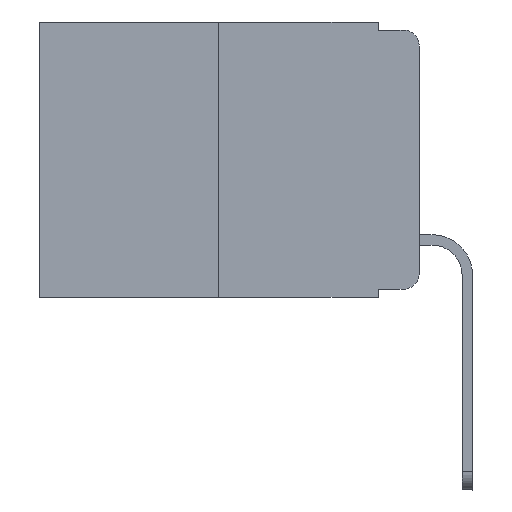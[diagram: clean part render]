
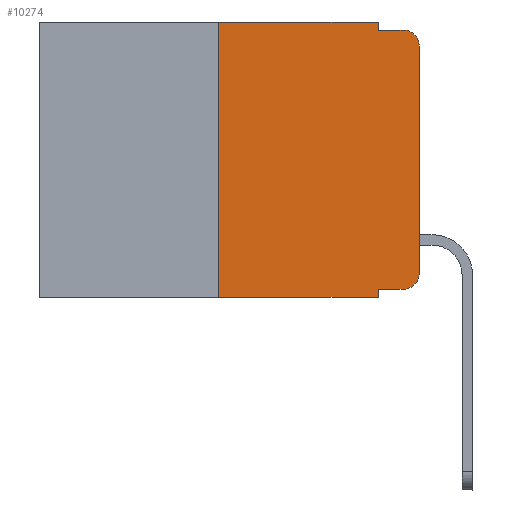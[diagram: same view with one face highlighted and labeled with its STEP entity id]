
A CAD part, left-side view. The second image highlights one B-rep face of the part: STEP entity #10274.
In plain terms, the highlighted planar face has unit normal (-1, 0, 0).
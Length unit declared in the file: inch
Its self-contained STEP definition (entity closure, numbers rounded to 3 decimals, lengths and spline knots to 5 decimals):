
#385 = EDGE_CURVE ( 'NONE', #6108, #2587, #17679, .T. ) ;
#498 = DIRECTION ( 'NONE',  ( 0., -1., 0. ) ) ;
#574 = DIRECTION ( 'NONE',  ( 0., 0., -1. ) ) ;
#698 = DIRECTION ( 'NONE',  ( 0., 0., -1. ) ) ;
#1213 = CARTESIAN_POINT ( 'NONE',  ( 0., 0.25, 0. ) ) ;
#1419 = LINE ( 'NONE', #10038, #11626 ) ;
#1794 = AXIS2_PLACEMENT_3D ( 'NONE', #13745, #10704, #574 ) ;
#1986 = FACE_OUTER_BOUND ( 'NONE', #2084, .T. ) ;
#2084 = EDGE_LOOP ( 'NONE', ( #8032, #12121, #10977, #15639, #12197, #11485, #10493, #4120, #3151, #17643 ) ) ;
#2191 = CARTESIAN_POINT ( 'NONE',  ( 0., 0.02, -0.313 ) ) ;
#2426 = AXIS2_PLACEMENT_3D ( 'NONE', #2191, #8846, #7192 ) ;
#2587 = VERTEX_POINT ( 'NONE', #17947 ) ;
#2642 = EDGE_CURVE ( 'NONE', #7393, #19901, #13010, .T. ) ;
#3125 = VERTEX_POINT ( 'NONE', #9799 ) ;
#3151 = ORIENTED_EDGE ( 'NONE', *, *, #16455, .T. ) ;
#3182 = CARTESIAN_POINT ( 'NONE',  ( 0., 0.051, 0. ) ) ;
#3537 = VECTOR ( 'NONE', #4506, 39.37008 ) ;
#3966 = VECTOR ( 'NONE', #498, 39.37008 ) ;
#4120 = ORIENTED_EDGE ( 'NONE', *, *, #11133, .F. ) ;
#4261 = CARTESIAN_POINT ( 'NONE',  ( 0., 0., -0.313 ) ) ;
#4506 = DIRECTION ( 'NONE',  ( 0., -1., 0. ) ) ;
#4751 = CARTESIAN_POINT ( 'NONE',  ( 0., 0.051, 0. ) ) ;
#4875 = CARTESIAN_POINT ( 'NONE',  ( 0., 0., 0. ) ) ;
#5364 = DIRECTION ( 'NONE',  ( 0., 0., -1. ) ) ;
#5461 = PLANE ( 'NONE',  #1794 ) ;
#5563 = VERTEX_POINT ( 'NONE', #12560 ) ;
#5573 = CIRCLE ( 'NONE', #2426, 0.02 ) ;
#5922 = CARTESIAN_POINT ( 'NONE',  ( 0., 0.25, -0.343 ) ) ;
#5993 = EDGE_CURVE ( 'NONE', #7393, #19561, #7523, .T. ) ;
#6108 = VERTEX_POINT ( 'NONE', #4261 ) ;
#6893 = CARTESIAN_POINT ( 'NONE',  ( 0., 0.02, -0.03 ) ) ;
#7192 = DIRECTION ( 'NONE',  ( 0., 0., -1. ) ) ;
#7393 = VERTEX_POINT ( 'NONE', #5922 ) ;
#7523 = LINE ( 'NONE', #1213, #11240 ) ;
#8032 = ORIENTED_EDGE ( 'NONE', *, *, #385, .T. ) ;
#8507 = CARTESIAN_POINT ( 'NONE',  ( 0., 0.051, -0.343 ) ) ;
#8748 = LINE ( 'NONE', #20549, #18710 ) ;
#8846 = DIRECTION ( 'NONE',  ( -1., 0., 0. ) ) ;
#9799 = CARTESIAN_POINT ( 'NONE',  ( 0., 0.051, -0.01 ) ) ;
#10038 = CARTESIAN_POINT ( 'NONE',  ( 0., 0.051, -0.333 ) ) ;
#10113 = LINE ( 'NONE', #16694, #3966 ) ;
#10274 = ADVANCED_FACE ( 'NONE', ( #1986 ), #5461, .F. ) ;
#10471 = VERTEX_POINT ( 'NONE', #20967 ) ;
#10493 = ORIENTED_EDGE ( 'NONE', *, *, #2642, .T. ) ;
#10535 = VECTOR ( 'NONE', #698, 39.37008 ) ;
#10611 = CARTESIAN_POINT ( 'NONE',  ( 0., 0.02, -0.333 ) ) ;
#10704 = DIRECTION ( 'NONE',  ( 1., 0., 0. ) ) ;
#10914 = EDGE_CURVE ( 'NONE', #14603, #3125, #16256, .T. ) ;
#10938 = AXIS2_PLACEMENT_3D ( 'NONE', #6893, #20119, #5364 ) ;
#10977 = ORIENTED_EDGE ( 'NONE', *, *, #17007, .F. ) ;
#11133 = EDGE_CURVE ( 'NONE', #10471, #19901, #15480, .T. ) ;
#11240 = VECTOR ( 'NONE', #15773, 39.37008 ) ;
#11401 = DIRECTION ( 'NONE',  ( 0., 0., -1. ) ) ;
#11485 = ORIENTED_EDGE ( 'NONE', *, *, #5993, .F. ) ;
#11533 = DIRECTION ( 'NONE',  ( 0., 0., 1. ) ) ;
#11626 = VECTOR ( 'NONE', #12978, 39.37008 ) ;
#12121 = ORIENTED_EDGE ( 'NONE', *, *, #12780, .T. ) ;
#12197 = ORIENTED_EDGE ( 'NONE', *, *, #19558, .F. ) ;
#12560 = CARTESIAN_POINT ( 'NONE',  ( 0., 0.02, -0.01 ) ) ;
#12780 = EDGE_CURVE ( 'NONE', #2587, #5563, #16458, .T. ) ;
#12978 = DIRECTION ( 'NONE',  ( 0., -1., 0. ) ) ;
#13010 = LINE ( 'NONE', #21309, #3537 ) ;
#13745 = CARTESIAN_POINT ( 'NONE',  ( 0., 0.473, 0. ) ) ;
#13753 = CARTESIAN_POINT ( 'NONE',  ( 0., 0.25, 0. ) ) ;
#13856 = DIRECTION ( 'NONE',  ( 0., -1., 0. ) ) ;
#14603 = VERTEX_POINT ( 'NONE', #3182 ) ;
#15480 = LINE ( 'NONE', #18713, #10535 ) ;
#15639 = ORIENTED_EDGE ( 'NONE', *, *, #10914, .F. ) ;
#15773 = DIRECTION ( 'NONE',  ( 0., 0., 1. ) ) ;
#16256 = LINE ( 'NONE', #4751, #18432 ) ;
#16455 = EDGE_CURVE ( 'NONE', #10471, #17413, #1419, .T. ) ;
#16458 = CIRCLE ( 'NONE', #10938, 0.02 ) ;
#16694 = CARTESIAN_POINT ( 'NONE',  ( 0., 0.051, -0.01 ) ) ;
#17007 = EDGE_CURVE ( 'NONE', #3125, #5563, #10113, .T. ) ;
#17413 = VERTEX_POINT ( 'NONE', #10611 ) ;
#17643 = ORIENTED_EDGE ( 'NONE', *, *, #21299, .T. ) ;
#17679 = LINE ( 'NONE', #4875, #18947 ) ;
#17947 = CARTESIAN_POINT ( 'NONE',  ( 0., 0., -0.03 ) ) ;
#18432 = VECTOR ( 'NONE', #11401, 39.37008 ) ;
#18710 = VECTOR ( 'NONE', #13856, 39.37008 ) ;
#18713 = CARTESIAN_POINT ( 'NONE',  ( 0., 0.051, 0. ) ) ;
#18947 = VECTOR ( 'NONE', #11533, 39.37008 ) ;
#19558 = EDGE_CURVE ( 'NONE', #19561, #14603, #8748, .T. ) ;
#19561 = VERTEX_POINT ( 'NONE', #13753 ) ;
#19901 = VERTEX_POINT ( 'NONE', #8507 ) ;
#20119 = DIRECTION ( 'NONE',  ( -1., 0., 0. ) ) ;
#20549 = CARTESIAN_POINT ( 'NONE',  ( 0., 0.473, 0. ) ) ;
#20967 = CARTESIAN_POINT ( 'NONE',  ( 0., 0.051, -0.333 ) ) ;
#21299 = EDGE_CURVE ( 'NONE', #17413, #6108, #5573, .T. ) ;
#21309 = CARTESIAN_POINT ( 'NONE',  ( 0., 0.473, -0.343 ) ) ;
